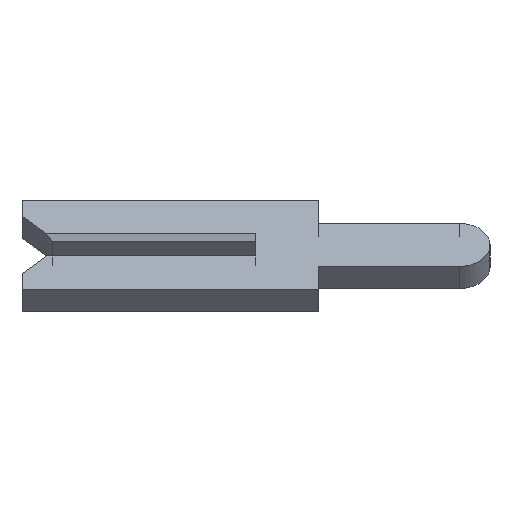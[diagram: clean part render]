
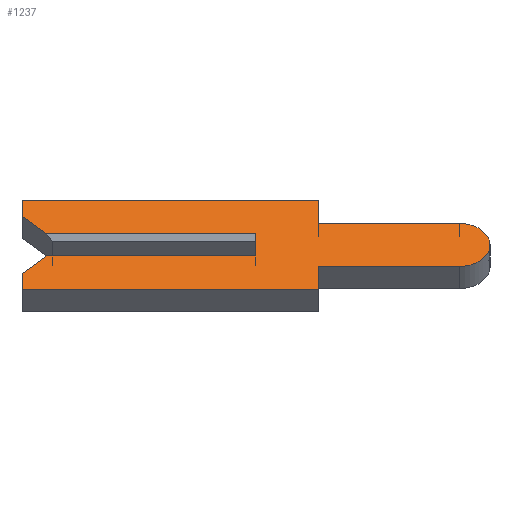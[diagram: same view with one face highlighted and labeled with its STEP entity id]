
A CAD part, left-side view. The second image highlights one B-rep face of the part: STEP entity #1237.
In plain terms, the highlighted face is planar.
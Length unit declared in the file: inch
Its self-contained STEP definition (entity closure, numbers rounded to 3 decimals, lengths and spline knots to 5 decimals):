
#18 = DIRECTION ( 'NONE',  ( 0., -1., 0. ) ) ;
#22 = LINE ( 'NONE', #1377, #768 ) ;
#30 = CARTESIAN_POINT ( 'NONE',  ( -0.01, -0.04, -0.04 ) ) ;
#39 = CARTESIAN_POINT ( 'NONE',  ( -0.01, -0.04, 0.04 ) ) ;
#44 = EDGE_CURVE ( 'NONE', #2103, #1670, #1930, .T. ) ;
#55 = ORIENTED_EDGE ( 'NONE', *, *, #1269, .F. ) ;
#62 = VECTOR ( 'NONE', #806, 39.37008 ) ;
#64 = VERTEX_POINT ( 'NONE', #1090 ) ;
#92 = VECTOR ( 'NONE', #463, 39.37008 ) ;
#97 = CARTESIAN_POINT ( 'NONE',  ( -0.01, -0.1305, -0.01 ) ) ;
#111 = ORIENTED_EDGE ( 'NONE', *, *, #2079, .F. ) ;
#119 = ORIENTED_EDGE ( 'NONE', *, *, #1816, .F. ) ;
#145 = VECTOR ( 'NONE', #632, 39.37008 ) ;
#184 = FACE_OUTER_BOUND ( 'NONE', #1312, .T. ) ;
#191 = ORIENTED_EDGE ( 'NONE', *, *, #297, .T. ) ;
#205 = VECTOR ( 'NONE', #1406, 39.37008 ) ;
#229 = VECTOR ( 'NONE', #389, 39.37008 ) ;
#230 = EDGE_CURVE ( 'NONE', #1768, #1014, #1984, .T. ) ;
#249 = DIRECTION ( 'NONE',  ( 0., 0., 1. ) ) ;
#262 = AXIS2_PLACEMENT_3D ( 'NONE', #1458, #920, #1780 ) ;
#285 = DIRECTION ( 'NONE',  ( 0., -1., 0. ) ) ;
#297 = EDGE_CURVE ( 'NONE', #383, #64, #1079, .T. ) ;
#322 = ORIENTED_EDGE ( 'NONE', *, *, #1694, .F. ) ;
#361 = PLANE ( 'NONE',  #593 ) ;
#383 = VERTEX_POINT ( 'NONE', #1471 ) ;
#385 = EDGE_CURVE ( 'NONE', #383, #2071, #1216, .T. ) ;
#389 = DIRECTION ( 'NONE',  ( 0., -1., 0. ) ) ;
#400 = ORIENTED_EDGE ( 'NONE', *, *, #385, .F. ) ;
#412 = LINE ( 'NONE', #1820, #1865 ) ;
#416 = EDGE_CURVE ( 'NONE', #1014, #64, #1846, .T. ) ;
#463 = DIRECTION ( 'NONE',  ( 0., 0., 1. ) ) ;
#487 = VERTEX_POINT ( 'NONE', #2031 ) ;
#515 = VERTEX_POINT ( 'NONE', #2048 ) ;
#518 = CARTESIAN_POINT ( 'NONE',  ( -0.01, -0.1305, 0. ) ) ;
#540 = DIRECTION ( 'NONE',  ( 0., 1., 0. ) ) ;
#571 = VECTOR ( 'NONE', #285, 39.37008 ) ;
#589 = CARTESIAN_POINT ( 'NONE',  ( -0.01, -0.1305, 0.0195 ) ) ;
#593 = AXIS2_PLACEMENT_3D ( 'NONE', #518, #695, #1383 ) ;
#632 = DIRECTION ( 'NONE',  ( 0., -1., 0. ) ) ;
#645 = VERTEX_POINT ( 'NONE', #1344 ) ;
#688 = LINE ( 'NONE', #1426, #1252 ) ;
#695 = DIRECTION ( 'NONE',  ( 1., 0., 0. ) ) ;
#719 = CARTESIAN_POINT ( 'NONE',  ( -0.01, -0.04, -0.0195 ) ) ;
#726 = CARTESIAN_POINT ( 'NONE',  ( -0.01, -0.1305, -0.0195 ) ) ;
#768 = VECTOR ( 'NONE', #18, 39.37008 ) ;
#780 = ORIENTED_EDGE ( 'NONE', *, *, #1901, .F. ) ;
#806 = DIRECTION ( 'NONE',  ( 0., 0.707, 0.707 ) ) ;
#821 = ORIENTED_EDGE ( 'NONE', *, *, #1339, .F. ) ;
#828 = VECTOR ( 'NONE', #1279, 39.37008 ) ;
#860 = ORIENTED_EDGE ( 'NONE', *, *, #44, .F. ) ;
#862 = CARTESIAN_POINT ( 'NONE',  ( -0.01, 0.15, -0.026 ) ) ;
#903 = CARTESIAN_POINT ( 'NONE',  ( -0.01, -0.04, 0.0195 ) ) ;
#914 = CARTESIAN_POINT ( 'NONE',  ( -0.01, 0.134, -0.01 ) ) ;
#920 = DIRECTION ( 'NONE',  ( 1., 0., 0. ) ) ;
#939 = DIRECTION ( 'NONE',  ( 0., 0., -1. ) ) ;
#961 = EDGE_CURVE ( 'NONE', #1710, #1709, #22, .T. ) ;
#962 = VERTEX_POINT ( 'NONE', #862 ) ;
#1014 = VERTEX_POINT ( 'NONE', #1015 ) ;
#1015 = CARTESIAN_POINT ( 'NONE',  ( -0.01, 0., -0.01 ) ) ;
#1035 = VECTOR ( 'NONE', #540, 39.37008 ) ;
#1054 = CARTESIAN_POINT ( 'NONE',  ( -0.01, 0.1305, -0.0065 ) ) ;
#1079 = LINE ( 'NONE', #1839, #571 ) ;
#1087 = VECTOR ( 'NONE', #939, 39.37008 ) ;
#1090 = CARTESIAN_POINT ( 'NONE',  ( -0.01, 0., 0.01 ) ) ;
#1124 = CARTESIAN_POINT ( 'NONE',  ( -0.01, 0.15, 0.026 ) ) ;
#1151 = CARTESIAN_POINT ( 'NONE',  ( -0.01, 0.1305, 0.0065 ) ) ;
#1216 = LINE ( 'NONE', #1151, #62 ) ;
#1237 = ADVANCED_FACE ( 'NONE', ( #184 ), #361, .F. ) ;
#1252 = VECTOR ( 'NONE', #2119, 39.37008 ) ;
#1267 = ORIENTED_EDGE ( 'NONE', *, *, #416, .F. ) ;
#1269 = EDGE_CURVE ( 'NONE', #1564, #645, #1284, .T. ) ;
#1279 = DIRECTION ( 'NONE',  ( 0., 0., 1. ) ) ;
#1284 = LINE ( 'NONE', #30, #1973 ) ;
#1307 = EDGE_CURVE ( 'NONE', #645, #515, #2056, .T. ) ;
#1312 = EDGE_LOOP ( 'NONE', ( #191, #1267, #2098, #821, #111, #1783, #55, #2180, #860, #322, #119, #1981, #780, #400 ) ) ;
#1339 = EDGE_CURVE ( 'NONE', #962, #1768, #1581, .T. ) ;
#1344 = CARTESIAN_POINT ( 'NONE',  ( -0.01, -0.04, -0.04 ) ) ;
#1377 = CARTESIAN_POINT ( 'NONE',  ( -0.01, 0.15, 0.04 ) ) ;
#1383 = DIRECTION ( 'NONE',  ( 0., 0., -1. ) ) ;
#1406 = DIRECTION ( 'NONE',  ( 0., -0.707, 0.707 ) ) ;
#1413 = CARTESIAN_POINT ( 'NONE',  ( -0.01, 0.15, -0.04 ) ) ;
#1426 = CARTESIAN_POINT ( 'NONE',  ( -0.01, -0.04, -0.0195 ) ) ;
#1456 = CARTESIAN_POINT ( 'NONE',  ( -0.01, -0.04, 0.04 ) ) ;
#1458 = CARTESIAN_POINT ( 'NONE',  ( -0.01, -0.1305, 0. ) ) ;
#1459 = EDGE_CURVE ( 'NONE', #1670, #1564, #688, .T. ) ;
#1471 = CARTESIAN_POINT ( 'NONE',  ( -0.01, 0.134, 0.01 ) ) ;
#1564 = VERTEX_POINT ( 'NONE', #719 ) ;
#1581 = LINE ( 'NONE', #1054, #205 ) ;
#1604 = CARTESIAN_POINT ( 'NONE',  ( -0.01, 0.15, 0.04 ) ) ;
#1646 = CARTESIAN_POINT ( 'NONE',  ( -0.01, 0., 0.0065 ) ) ;
#1656 = LINE ( 'NONE', #903, #229 ) ;
#1670 = VERTEX_POINT ( 'NONE', #726 ) ;
#1694 = EDGE_CURVE ( 'NONE', #487, #2103, #1656, .T. ) ;
#1698 = LINE ( 'NONE', #1977, #828 ) ;
#1709 = VERTEX_POINT ( 'NONE', #39 ) ;
#1710 = VERTEX_POINT ( 'NONE', #1604 ) ;
#1768 = VERTEX_POINT ( 'NONE', #914 ) ;
#1780 = DIRECTION ( 'NONE',  ( 0., 0., -1. ) ) ;
#1783 = ORIENTED_EDGE ( 'NONE', *, *, #1307, .F. ) ;
#1816 = EDGE_CURVE ( 'NONE', #1709, #487, #2052, .T. ) ;
#1820 = CARTESIAN_POINT ( 'NONE',  ( -0.01, 0.15, 0.026 ) ) ;
#1839 = CARTESIAN_POINT ( 'NONE',  ( -0.01, 0.15, 0.01 ) ) ;
#1846 = LINE ( 'NONE', #1646, #92 ) ;
#1865 = VECTOR ( 'NONE', #249, 39.37008 ) ;
#1901 = EDGE_CURVE ( 'NONE', #2071, #1710, #412, .T. ) ;
#1902 = DIRECTION ( 'NONE',  ( 0., 0., -1. ) ) ;
#1930 = CIRCLE ( 'NONE', #262, 0.0195 ) ;
#1973 = VECTOR ( 'NONE', #1902, 39.37008 ) ;
#1977 = CARTESIAN_POINT ( 'NONE',  ( -0.01, 0.15, -0.026 ) ) ;
#1981 = ORIENTED_EDGE ( 'NONE', *, *, #961, .F. ) ;
#1984 = LINE ( 'NONE', #97, #145 ) ;
#2031 = CARTESIAN_POINT ( 'NONE',  ( -0.01, -0.04, 0.0195 ) ) ;
#2048 = CARTESIAN_POINT ( 'NONE',  ( -0.01, 0.15, -0.04 ) ) ;
#2052 = LINE ( 'NONE', #1456, #1087 ) ;
#2056 = LINE ( 'NONE', #1413, #1035 ) ;
#2071 = VERTEX_POINT ( 'NONE', #1124 ) ;
#2079 = EDGE_CURVE ( 'NONE', #515, #962, #1698, .T. ) ;
#2098 = ORIENTED_EDGE ( 'NONE', *, *, #230, .F. ) ;
#2103 = VERTEX_POINT ( 'NONE', #589 ) ;
#2119 = DIRECTION ( 'NONE',  ( 0., 1., 0. ) ) ;
#2180 = ORIENTED_EDGE ( 'NONE', *, *, #1459, .F. ) ;
